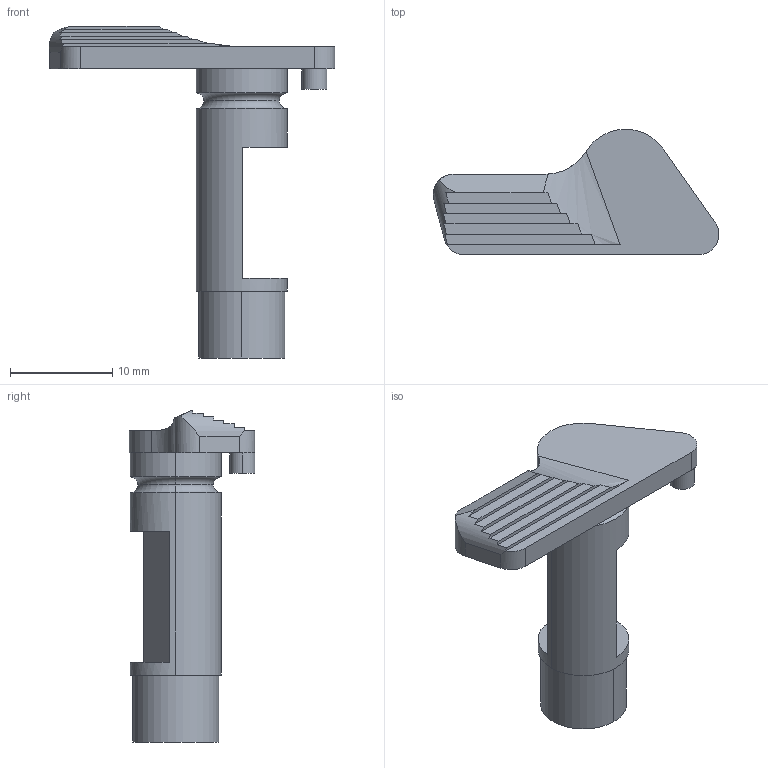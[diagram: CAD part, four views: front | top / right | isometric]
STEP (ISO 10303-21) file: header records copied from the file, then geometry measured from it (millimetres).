
FILE_DESCRIPTION (( 'STEP AP214' ), '1' );
FILE_NAME ('Takedown Lever.step', '2014-07-30T19:47:06', ( 'WarFairy' ), ( '' ), 'SwSTEP 2.0', 'SolidWorks 2013', '' );
FILE_SCHEMA (( 'AUTOMOTIVE_DESIGN' ));
Length unit declared in the file: millimetre
Products named in the file (1): Takedown Lever
Bounding box: 27.94 x 12.27 x 32.47 mm (x, y, z)
Volume: 1846.5 mm3; surface area: 1459.4 mm2
Topology: 1 solids, 1 shells, 45 faces, 114 edges, 73 vertices
Faces by surface type: plane 26, cylinder 14, torus 4, bspline 1
Entity records: 1411 total; most frequent: CARTESIAN_POINT 293, DIRECTION 232, ORIENTED_EDGE 228, EDGE_CURVE 114, AXIS2_PLACEMENT_3D 86, VERTEX_POINT 73, VECTOR 60, LINE 60
